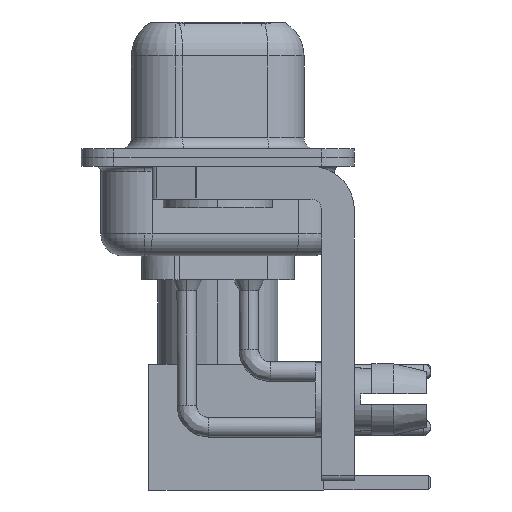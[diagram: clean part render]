
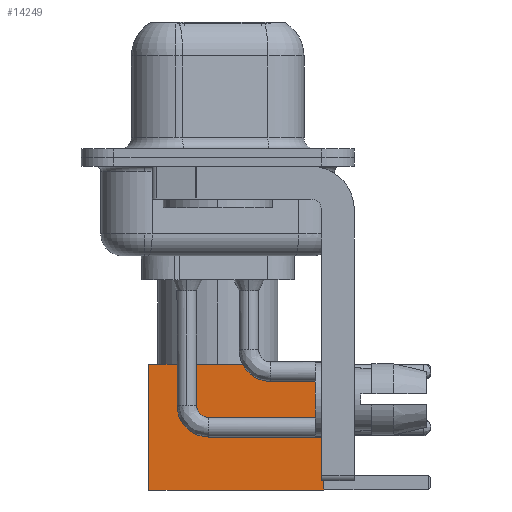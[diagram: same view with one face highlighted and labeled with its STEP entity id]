
A CAD part, left-side view. The second image highlights one B-rep face of the part: STEP entity #14249.
In plain terms, the highlighted face is planar.
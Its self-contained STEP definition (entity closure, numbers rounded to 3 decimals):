
#119 = CARTESIAN_POINT ( 'NONE',  ( 0., 2.875, 8. ) ) ;
#1955 = CARTESIAN_POINT ( 'NONE',  ( 2.875, 2.875, 8. ) ) ;
#2003 = VECTOR ( 'NONE', #5035, 1000. ) ;
#2320 = CARTESIAN_POINT ( 'NONE',  ( 2.875, 2.875, 0. ) ) ;
#2451 = EDGE_CURVE ( 'NONE', #21624, #13830, #3492, .T. ) ;
#2860 = ORIENTED_EDGE ( 'NONE', *, *, #9357, .F. ) ;
#3492 = LINE ( 'NONE', #20113, #18256 ) ;
#3559 = DIRECTION ( 'NONE',  ( -1., 0., 0. ) ) ;
#5035 = DIRECTION ( 'NONE',  ( 0., 0., -1. ) ) ;
#5772 = CARTESIAN_POINT ( 'NONE',  ( -2.875, 2.875, 0. ) ) ;
#5972 = PLANE ( 'NONE',  #19005 ) ;
#7598 = EDGE_CURVE ( 'NONE', #15991, #13830, #15066, .T. ) ;
#7811 = DIRECTION ( 'NONE',  ( 0., 0., 1. ) ) ;
#7954 = EDGE_CURVE ( 'NONE', #9402, #21624, #10525, .T. ) ;
#9211 = DIRECTION ( 'NONE',  ( -1., 0., 0. ) ) ;
#9357 = EDGE_CURVE ( 'NONE', #9402, #15991, #10764, .T. ) ;
#9402 = VERTEX_POINT ( 'NONE', #1955 ) ;
#10432 = CARTESIAN_POINT ( 'NONE',  ( -2.875, 2.875, 8. ) ) ;
#10525 = LINE ( 'NONE', #21789, #2003 ) ;
#10764 = LINE ( 'NONE', #119, #14892 ) ;
#11232 = FACE_OUTER_BOUND ( 'NONE', #12577, .T. ) ;
#11395 = CARTESIAN_POINT ( 'NONE',  ( 2.875, 2.875, 0. ) ) ;
#12577 = EDGE_LOOP ( 'NONE', ( #14560, #16866, #17000, #2860 ) ) ;
#13070 = DIRECTION ( 'NONE',  ( 0., 1., 0. ) ) ;
#13830 = VERTEX_POINT ( 'NONE', #22650 ) ;
#14249 = ADVANCED_FACE ( 'NONE', ( #11232 ), #5972, .T. ) ;
#14560 = ORIENTED_EDGE ( 'NONE', *, *, #7954, .T. ) ;
#14700 = DIRECTION ( 'NONE',  ( 0., 0., -1. ) ) ;
#14892 = VECTOR ( 'NONE', #3559, 1000. ) ;
#15066 = LINE ( 'NONE', #5772, #18413 ) ;
#15991 = VERTEX_POINT ( 'NONE', #10432 ) ;
#16866 = ORIENTED_EDGE ( 'NONE', *, *, #2451, .T. ) ;
#17000 = ORIENTED_EDGE ( 'NONE', *, *, #7598, .F. ) ;
#18256 = VECTOR ( 'NONE', #9211, 1000. ) ;
#18413 = VECTOR ( 'NONE', #14700, 1000. ) ;
#19005 = AXIS2_PLACEMENT_3D ( 'NONE', #2320, #13070, #7811 ) ;
#20113 = CARTESIAN_POINT ( 'NONE',  ( 0., 2.875, 0. ) ) ;
#21624 = VERTEX_POINT ( 'NONE', #11395 ) ;
#21789 = CARTESIAN_POINT ( 'NONE',  ( 2.875, 2.875, 0. ) ) ;
#22650 = CARTESIAN_POINT ( 'NONE',  ( -2.875, 2.875, 0. ) ) ;
